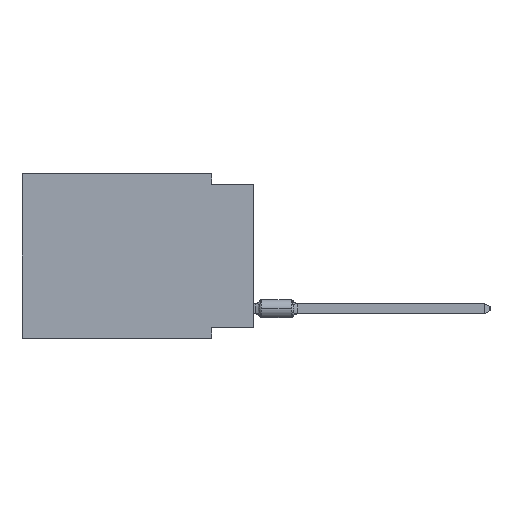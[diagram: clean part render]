
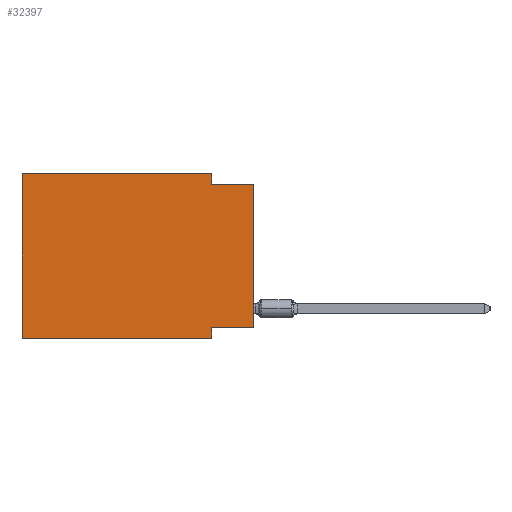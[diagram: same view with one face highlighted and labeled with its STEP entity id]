
A CAD part, left-side view. The second image highlights one B-rep face of the part: STEP entity #32397.
In plain terms, the highlighted planar face has unit normal (-1, 0, 0).
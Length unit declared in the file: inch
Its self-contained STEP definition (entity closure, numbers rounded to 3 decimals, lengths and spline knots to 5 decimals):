
#771 = CARTESIAN_POINT ( 'NONE',  ( 0., 0., -0.025 ) ) ;
#1522 = EDGE_CURVE ( 'NONE', #25202, #20825, #20714, .T. ) ;
#3493 = EDGE_CURVE ( 'NONE', #39750, #3886, #19500, .T. ) ;
#3535 = ORIENTED_EDGE ( 'NONE', *, *, #3493, .F. ) ;
#3886 = VERTEX_POINT ( 'NONE', #21269 ) ;
#5445 = VERTEX_POINT ( 'NONE', #52882 ) ;
#7298 = CARTESIAN_POINT ( 'NONE',  ( 0., 0.1, -0.39 ) ) ;
#8715 = DIRECTION ( 'NONE',  ( 0., 0., -1. ) ) ;
#9214 = DIRECTION ( 'NONE',  ( 0., -1., 0. ) ) ;
#9780 = VECTOR ( 'NONE', #38627, 39.37008 ) ;
#10052 = CARTESIAN_POINT ( 'NONE',  ( 0., 0.55, -0.39 ) ) ;
#10448 = VECTOR ( 'NONE', #9214, 39.37008 ) ;
#12287 = FACE_OUTER_BOUND ( 'NONE', #40951, .T. ) ;
#12502 = VECTOR ( 'NONE', #29804, 39.37008 ) ;
#12970 = ORIENTED_EDGE ( 'NONE', *, *, #17520, .T. ) ;
#13429 = DIRECTION ( 'NONE',  ( 0., 0., -1. ) ) ;
#14030 = EDGE_CURVE ( 'NONE', #5445, #40502, #38380, .T. ) ;
#14328 = VECTOR ( 'NONE', #35552, 39.37008 ) ;
#16884 = EDGE_CURVE ( 'NONE', #47507, #20051, #30187, .T. ) ;
#17227 = AXIS2_PLACEMENT_3D ( 'NONE', #20711, #41691, #8715 ) ;
#17520 = EDGE_CURVE ( 'NONE', #39750, #40502, #18640, .T. ) ;
#18640 = LINE ( 'NONE', #31483, #14328 ) ;
#18884 = VECTOR ( 'NONE', #22119, 39.37008 ) ;
#19500 = LINE ( 'NONE', #53304, #29457 ) ;
#20051 = VERTEX_POINT ( 'NONE', #7298 ) ;
#20451 = DIRECTION ( 'NONE',  ( 0., -1., 0. ) ) ;
#20711 = CARTESIAN_POINT ( 'NONE',  ( 0., 0.55, 0. ) ) ;
#20714 = LINE ( 'NONE', #49071, #37689 ) ;
#20825 = VERTEX_POINT ( 'NONE', #53035 ) ;
#21269 = CARTESIAN_POINT ( 'NONE',  ( 0., 0.1, -0.365 ) ) ;
#21605 = LINE ( 'NONE', #26229, #12502 ) ;
#22052 = ORIENTED_EDGE ( 'NONE', *, *, #14030, .F. ) ;
#22119 = DIRECTION ( 'NONE',  ( 0., 0., -1. ) ) ;
#22132 = LINE ( 'NONE', #26482, #30012 ) ;
#25202 = VERTEX_POINT ( 'NONE', #50685 ) ;
#26229 = CARTESIAN_POINT ( 'NONE',  ( 0., 0.55, 0. ) ) ;
#26482 = CARTESIAN_POINT ( 'NONE',  ( 0., 0.1, 0. ) ) ;
#26574 = ORIENTED_EDGE ( 'NONE', *, *, #50248, .F. ) ;
#27538 = ORIENTED_EDGE ( 'NONE', *, *, #1522, .F. ) ;
#29444 = PLANE ( 'NONE',  #17227 ) ;
#29457 = VECTOR ( 'NONE', #52757, 39.37008 ) ;
#29804 = DIRECTION ( 'NONE',  ( 0., 0., 1. ) ) ;
#30012 = VECTOR ( 'NONE', #13429, 39.37008 ) ;
#30187 = LINE ( 'NONE', #42968, #9780 ) ;
#30372 = EDGE_CURVE ( 'NONE', #20825, #5445, #22132, .T. ) ;
#31483 = CARTESIAN_POINT ( 'NONE',  ( 0., 0., 0. ) ) ;
#32397 = ADVANCED_FACE ( 'NONE', ( #12287 ), #29444, .F. ) ;
#35552 = DIRECTION ( 'NONE',  ( 0., 0., 1. ) ) ;
#37641 = CARTESIAN_POINT ( 'NONE',  ( 0., 0., -0.365 ) ) ;
#37689 = VECTOR ( 'NONE', #20451, 39.37008 ) ;
#38380 = LINE ( 'NONE', #771, #10448 ) ;
#38627 = DIRECTION ( 'NONE',  ( 0., -1., 0. ) ) ;
#38741 = LINE ( 'NONE', #46642, #18884 ) ;
#39750 = VERTEX_POINT ( 'NONE', #37641 ) ;
#39863 = ORIENTED_EDGE ( 'NONE', *, *, #30372, .F. ) ;
#40395 = EDGE_CURVE ( 'NONE', #47507, #25202, #21605, .T. ) ;
#40502 = VERTEX_POINT ( 'NONE', #48284 ) ;
#40951 = EDGE_LOOP ( 'NONE', ( #12970, #22052, #39863, #27538, #47173, #41884, #26574, #3535 ) ) ;
#41691 = DIRECTION ( 'NONE',  ( 1., 0., 0. ) ) ;
#41884 = ORIENTED_EDGE ( 'NONE', *, *, #16884, .T. ) ;
#42968 = CARTESIAN_POINT ( 'NONE',  ( 0., 0.55, -0.39 ) ) ;
#46642 = CARTESIAN_POINT ( 'NONE',  ( 0., 0.1, -0.39 ) ) ;
#47173 = ORIENTED_EDGE ( 'NONE', *, *, #40395, .F. ) ;
#47507 = VERTEX_POINT ( 'NONE', #10052 ) ;
#48284 = CARTESIAN_POINT ( 'NONE',  ( 0., 0., -0.025 ) ) ;
#49071 = CARTESIAN_POINT ( 'NONE',  ( 0., 0.55, 0. ) ) ;
#50248 = EDGE_CURVE ( 'NONE', #3886, #20051, #38741, .T. ) ;
#50685 = CARTESIAN_POINT ( 'NONE',  ( 0., 0.55, 0. ) ) ;
#52757 = DIRECTION ( 'NONE',  ( 0., 1., 0. ) ) ;
#52882 = CARTESIAN_POINT ( 'NONE',  ( 0., 0.1, -0.025 ) ) ;
#53035 = CARTESIAN_POINT ( 'NONE',  ( 0., 0.1, 0. ) ) ;
#53304 = CARTESIAN_POINT ( 'NONE',  ( 0., 0., -0.365 ) ) ;
